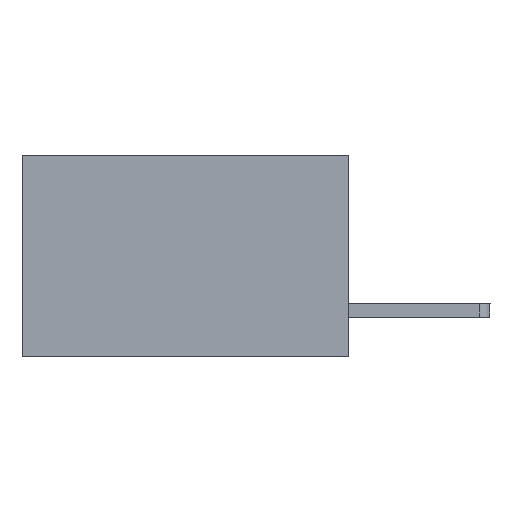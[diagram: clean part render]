
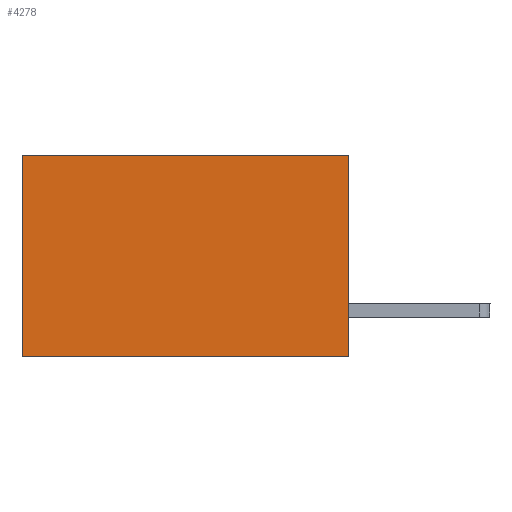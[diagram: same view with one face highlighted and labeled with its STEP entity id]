
A CAD part, left-side view. The second image highlights one B-rep face of the part: STEP entity #4278.
In plain terms, the highlighted planar face has unit normal (-1, 0, 0).
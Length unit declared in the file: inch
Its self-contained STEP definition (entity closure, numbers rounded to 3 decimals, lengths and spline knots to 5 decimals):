
#531 = VECTOR ( 'NONE', #8302, 39.37008 ) ;
#1087 = VECTOR ( 'NONE', #11665, 39.37008 ) ;
#1474 = CARTESIAN_POINT ( 'NONE',  ( 0.298, 0.6, -0.37 ) ) ;
#3081 = VERTEX_POINT ( 'NONE', #7471 ) ;
#3273 = CARTESIAN_POINT ( 'NONE',  ( 0.298, 0., 0. ) ) ;
#3657 = VECTOR ( 'NONE', #9783, 39.37008 ) ;
#4207 = PLANE ( 'NONE',  #4520 ) ;
#4278 = ADVANCED_FACE ( 'NONE', ( #6935 ), #4207, .F. ) ;
#4520 = AXIS2_PLACEMENT_3D ( 'NONE', #7647, #10366, #4933 ) ;
#4768 = EDGE_CURVE ( 'NONE', #6340, #3081, #6086, .T. ) ;
#4933 = DIRECTION ( 'NONE',  ( 0., 0., -1. ) ) ;
#5606 = ORIENTED_EDGE ( 'NONE', *, *, #8330, .F. ) ;
#6015 = VECTOR ( 'NONE', #10289, 39.37008 ) ;
#6086 = LINE ( 'NONE', #10082, #3657 ) ;
#6340 = VERTEX_POINT ( 'NONE', #3273 ) ;
#6634 = ORIENTED_EDGE ( 'NONE', *, *, #11162, .F. ) ;
#6769 = CARTESIAN_POINT ( 'NONE',  ( 0.298, 0., -0.37 ) ) ;
#6935 = FACE_OUTER_BOUND ( 'NONE', #8793, .T. ) ;
#6972 = ORIENTED_EDGE ( 'NONE', *, *, #8051, .T. ) ;
#7126 = VERTEX_POINT ( 'NONE', #1474 ) ;
#7471 = CARTESIAN_POINT ( 'NONE',  ( 0.298, 0.6, 0. ) ) ;
#7647 = CARTESIAN_POINT ( 'NONE',  ( 0.298, 0., 0. ) ) ;
#8051 = EDGE_CURVE ( 'NONE', #3081, #7126, #8686, .T. ) ;
#8302 = DIRECTION ( 'NONE',  ( 0., 1., 0. ) ) ;
#8330 = EDGE_CURVE ( 'NONE', #6340, #11655, #11367, .T. ) ;
#8686 = LINE ( 'NONE', #11788, #1087 ) ;
#8793 = EDGE_LOOP ( 'NONE', ( #6972, #6634, #5606, #9575 ) ) ;
#9575 = ORIENTED_EDGE ( 'NONE', *, *, #4768, .T. ) ;
#9783 = DIRECTION ( 'NONE',  ( 0., 1., 0. ) ) ;
#10082 = CARTESIAN_POINT ( 'NONE',  ( 0.298, 0., 0. ) ) ;
#10289 = DIRECTION ( 'NONE',  ( 0., 0., -1. ) ) ;
#10366 = DIRECTION ( 'NONE',  ( 1., 0., 0. ) ) ;
#10418 = CARTESIAN_POINT ( 'NONE',  ( 0.298, 0., 0. ) ) ;
#11036 = CARTESIAN_POINT ( 'NONE',  ( 0.298, 0., -0.37 ) ) ;
#11111 = LINE ( 'NONE', #11036, #531 ) ;
#11162 = EDGE_CURVE ( 'NONE', #11655, #7126, #11111, .T. ) ;
#11367 = LINE ( 'NONE', #10418, #6015 ) ;
#11655 = VERTEX_POINT ( 'NONE', #6769 ) ;
#11665 = DIRECTION ( 'NONE',  ( 0., 0., -1. ) ) ;
#11788 = CARTESIAN_POINT ( 'NONE',  ( 0.298, 0.6, 0. ) ) ;
